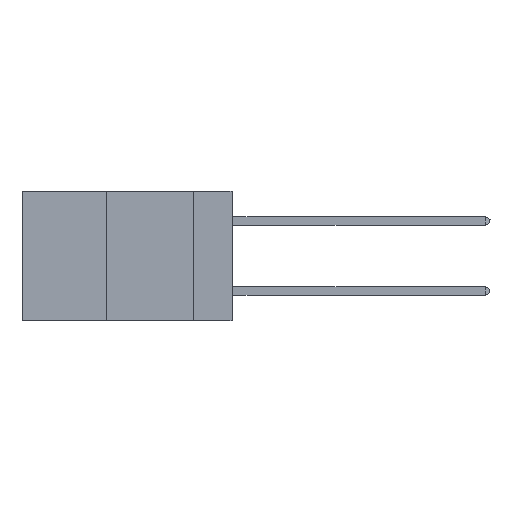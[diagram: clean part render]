
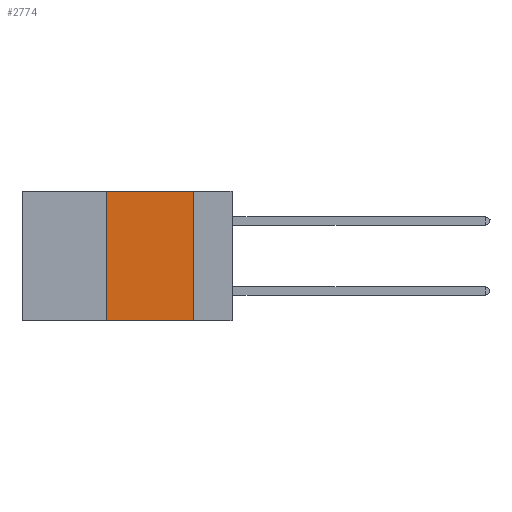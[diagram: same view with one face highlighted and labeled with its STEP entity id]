
A CAD part, left-side view. The second image highlights one B-rep face of the part: STEP entity #2774.
In plain terms, the highlighted planar face has unit normal (-1, 0, 0).
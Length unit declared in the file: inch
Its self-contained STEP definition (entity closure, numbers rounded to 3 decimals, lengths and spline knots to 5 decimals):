
#358 = PLANE ( 'NONE',  #7614 ) ;
#1240 = VECTOR ( 'NONE', #20006, 39.37008 ) ;
#1241 = VERTEX_POINT ( 'NONE', #18496 ) ;
#1364 = CARTESIAN_POINT ( 'NONE',  ( 0., 0.6, -0.37 ) ) ;
#1480 = DIRECTION ( 'NONE',  ( 0., -1., 0. ) ) ;
#2774 = ADVANCED_FACE ( 'NONE', ( #22702 ), #358, .F. ) ;
#3320 = VECTOR ( 'NONE', #17591, 39.37008 ) ;
#3875 = LINE ( 'NONE', #13788, #3320 ) ;
#4003 = LINE ( 'NONE', #13085, #4165 ) ;
#4165 = VECTOR ( 'NONE', #11368, 39.37008 ) ;
#7412 = VERTEX_POINT ( 'NONE', #17447 ) ;
#7614 = AXIS2_PLACEMENT_3D ( 'NONE', #11780, #21077, #17414 ) ;
#8501 = VERTEX_POINT ( 'NONE', #10536 ) ;
#9277 = ORIENTED_EDGE ( 'NONE', *, *, #19913, .F. ) ;
#9444 = ORIENTED_EDGE ( 'NONE', *, *, #11582, .F. ) ;
#10536 = CARTESIAN_POINT ( 'NONE',  ( 0., 0.36, 0. ) ) ;
#10703 = LINE ( 'NONE', #1364, #21855 ) ;
#11368 = DIRECTION ( 'NONE',  ( 0., 0., 1. ) ) ;
#11582 = EDGE_CURVE ( 'NONE', #8501, #7412, #3875, .T. ) ;
#11780 = CARTESIAN_POINT ( 'NONE',  ( 0., 0.6, 0. ) ) ;
#12431 = LINE ( 'NONE', #12545, #1240 ) ;
#12545 = CARTESIAN_POINT ( 'NONE',  ( 0., 0.11, 0. ) ) ;
#13085 = CARTESIAN_POINT ( 'NONE',  ( 0., 0.36, 0. ) ) ;
#13747 = VERTEX_POINT ( 'NONE', #17069 ) ;
#13788 = CARTESIAN_POINT ( 'NONE',  ( 0., 0.6, 0. ) ) ;
#14139 = EDGE_CURVE ( 'NONE', #7412, #1241, #12431, .T. ) ;
#14698 = EDGE_LOOP ( 'NONE', ( #17610, #9444, #9277, #19723 ) ) ;
#17069 = CARTESIAN_POINT ( 'NONE',  ( 0., 0.36, -0.37 ) ) ;
#17414 = DIRECTION ( 'NONE',  ( 0., 0., -1. ) ) ;
#17447 = CARTESIAN_POINT ( 'NONE',  ( 0., 0.11, 0. ) ) ;
#17591 = DIRECTION ( 'NONE',  ( 0., -1., 0. ) ) ;
#17610 = ORIENTED_EDGE ( 'NONE', *, *, #14139, .F. ) ;
#18496 = CARTESIAN_POINT ( 'NONE',  ( 0., 0.11, -0.37 ) ) ;
#19723 = ORIENTED_EDGE ( 'NONE', *, *, #22066, .T. ) ;
#19913 = EDGE_CURVE ( 'NONE', #13747, #8501, #4003, .T. ) ;
#20006 = DIRECTION ( 'NONE',  ( 0., 0., -1. ) ) ;
#21077 = DIRECTION ( 'NONE',  ( 1., 0., 0. ) ) ;
#21855 = VECTOR ( 'NONE', #1480, 39.37008 ) ;
#22066 = EDGE_CURVE ( 'NONE', #13747, #1241, #10703, .T. ) ;
#22702 = FACE_OUTER_BOUND ( 'NONE', #14698, .T. ) ;
